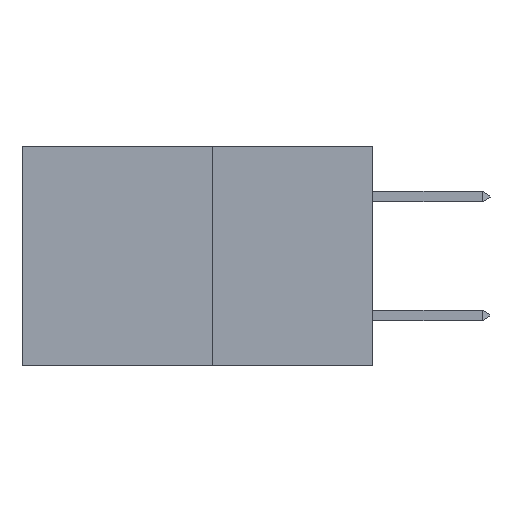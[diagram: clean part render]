
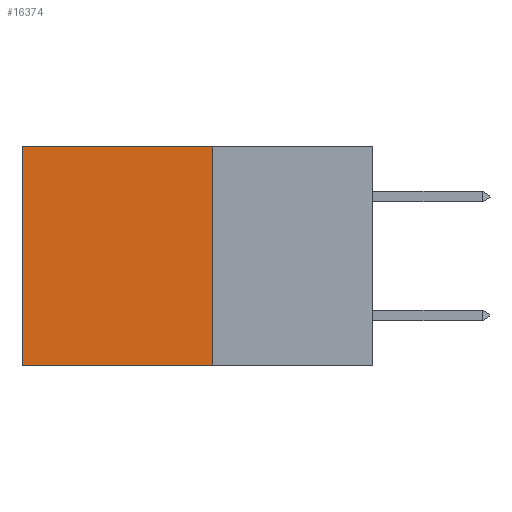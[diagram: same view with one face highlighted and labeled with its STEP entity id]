
A CAD part, left-side view. The second image highlights one B-rep face of the part: STEP entity #16374.
In plain terms, the highlighted planar face has unit normal (-1, 0, 0).
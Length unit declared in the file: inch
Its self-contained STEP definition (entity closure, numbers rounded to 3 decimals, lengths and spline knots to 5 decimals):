
#161 = ORIENTED_EDGE ( 'NONE', *, *, #10791, .T. ) ;
#207 = VECTOR ( 'NONE', #10505, 39.37008 ) ;
#874 = LINE ( 'NONE', #15715, #6899 ) ;
#2009 = ORIENTED_EDGE ( 'NONE', *, *, #7402, .F. ) ;
#2509 = CARTESIAN_POINT ( 'NONE',  ( 0.277, 0.59, -0.37 ) ) ;
#2650 = EDGE_CURVE ( 'NONE', #6978, #5002, #3676, .T. ) ;
#3676 = LINE ( 'NONE', #5915, #207 ) ;
#4516 = ORIENTED_EDGE ( 'NONE', *, *, #2650, .F. ) ;
#4986 = FACE_OUTER_BOUND ( 'NONE', #9962, .T. ) ;
#5002 = VERTEX_POINT ( 'NONE', #8871 ) ;
#5915 = CARTESIAN_POINT ( 'NONE',  ( 0.277, 0.27, -0.37 ) ) ;
#6118 = CARTESIAN_POINT ( 'NONE',  ( 0.277, 0.27, 0. ) ) ;
#6217 = DIRECTION ( 'NONE',  ( 0., 0., -1. ) ) ;
#6899 = VECTOR ( 'NONE', #8259, 39.37008 ) ;
#6978 = VERTEX_POINT ( 'NONE', #6118 ) ;
#7402 = EDGE_CURVE ( 'NONE', #5002, #11106, #10693, .T. ) ;
#7532 = VECTOR ( 'NONE', #13718, 39.37008 ) ;
#8259 = DIRECTION ( 'NONE',  ( 0., 0., -1. ) ) ;
#8871 = CARTESIAN_POINT ( 'NONE',  ( 0.277, 0.27, -0.37 ) ) ;
#9073 = ORIENTED_EDGE ( 'NONE', *, *, #9134, .T. ) ;
#9134 = EDGE_CURVE ( 'NONE', #6978, #14362, #14214, .T. ) ;
#9828 = AXIS2_PLACEMENT_3D ( 'NONE', #12470, #13742, #6217 ) ;
#9962 = EDGE_LOOP ( 'NONE', ( #161, #2009, #4516, #9073 ) ) ;
#10286 = VECTOR ( 'NONE', #13249, 39.37008 ) ;
#10505 = DIRECTION ( 'NONE',  ( 0., 0., -1. ) ) ;
#10693 = LINE ( 'NONE', #11963, #10286 ) ;
#10791 = EDGE_CURVE ( 'NONE', #14362, #11106, #874, .T. ) ;
#11106 = VERTEX_POINT ( 'NONE', #2509 ) ;
#11180 = PLANE ( 'NONE',  #9828 ) ;
#11963 = CARTESIAN_POINT ( 'NONE',  ( 0.277, 0.27, -0.37 ) ) ;
#12470 = CARTESIAN_POINT ( 'NONE',  ( 0.277, 0.27, -0.37 ) ) ;
#12973 = CARTESIAN_POINT ( 'NONE',  ( 0.277, 0.59, 0. ) ) ;
#13249 = DIRECTION ( 'NONE',  ( 0., 1., 0. ) ) ;
#13718 = DIRECTION ( 'NONE',  ( 0., 1., 0. ) ) ;
#13742 = DIRECTION ( 'NONE',  ( 1., 0., 0. ) ) ;
#14214 = LINE ( 'NONE', #14974, #7532 ) ;
#14362 = VERTEX_POINT ( 'NONE', #12973 ) ;
#14974 = CARTESIAN_POINT ( 'NONE',  ( 0.277, 0.27, 0. ) ) ;
#15715 = CARTESIAN_POINT ( 'NONE',  ( 0.277, 0.59, -0.37 ) ) ;
#16374 = ADVANCED_FACE ( 'NONE', ( #4986 ), #11180, .F. ) ;
